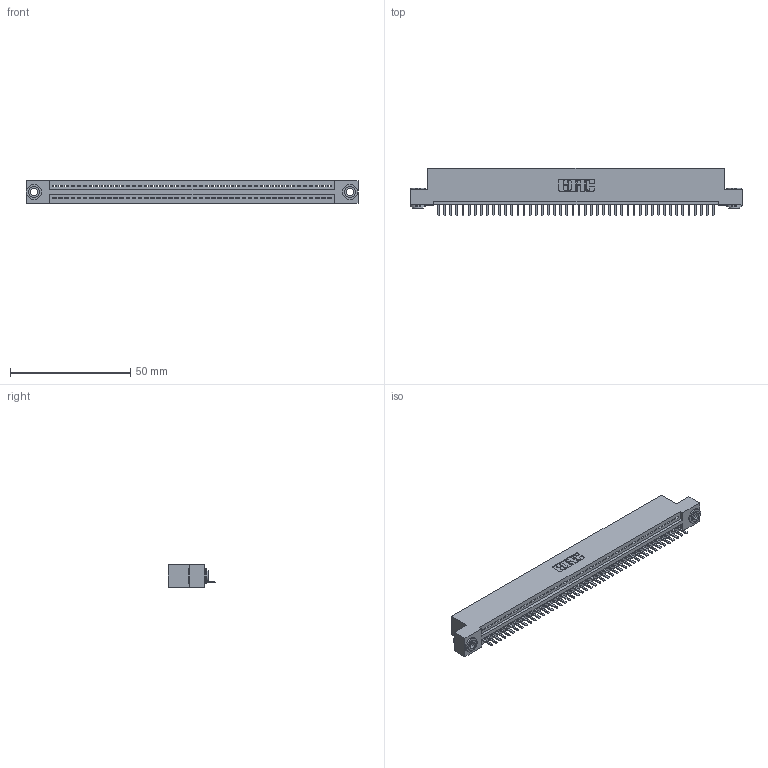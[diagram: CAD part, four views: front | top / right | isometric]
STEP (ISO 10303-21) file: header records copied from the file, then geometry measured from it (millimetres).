
FILE_DESCRIPTION (( 'STEP AP203' ), '1' );
FILE_NAME ('395-046-520-103.STEP', '2019-10-22T19:53:54', ( '' ), ( '' ), 'SwSTEP 2.0', 'SolidWorks 2016', '' );
FILE_SCHEMA (( 'CONFIG_CONTROL_DESIGN' ));
Length unit declared in the file: inch
Products named in the file (4): 345-292-001_345-293-120; 345-250-002_345-250-002-102; 395-046-520-103; 345 Part_Flush Mounting Lugs - 0.156 Dia-TH
Assembly tree (49 placements, depth 2):
  395-046-520-103
    345 Part_Flush Mounting Lugs - 0.156 Dia-TH
    345-292-001_345-293-120  x46
    345-250-002_345-250-002-102  x2
Bounding box: 138.05 x 19.68 x 9.4 mm (x, y, z)
Volume: 13031.9 mm3; surface area: 17154.2 mm2
Topology: 49 solids, 49 shells, 3016 faces, 8881 edges, 5794 vertices
Faces by surface type: plane 2022, cylinder 986, cone 8
Entity records: 34846 total; most frequent: CARTESIAN_POINT 6025, ORIENTED_EDGE 5986, DIRECTION 5275, EDGE_CURVE 2993, VECTOR 2649, LINE 2649, VERTEX_POINT 1990, AXIS2_PLACEMENT_3D 1313
